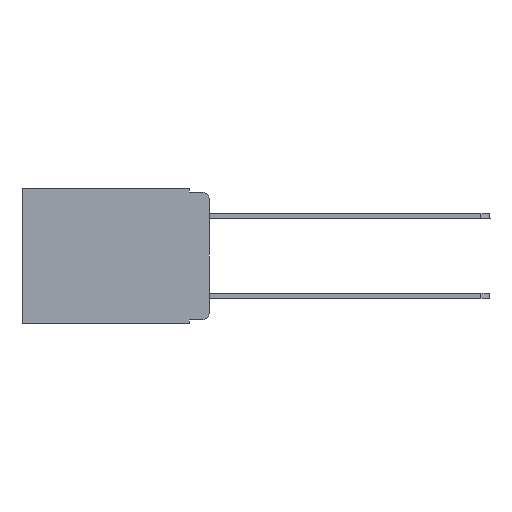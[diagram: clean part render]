
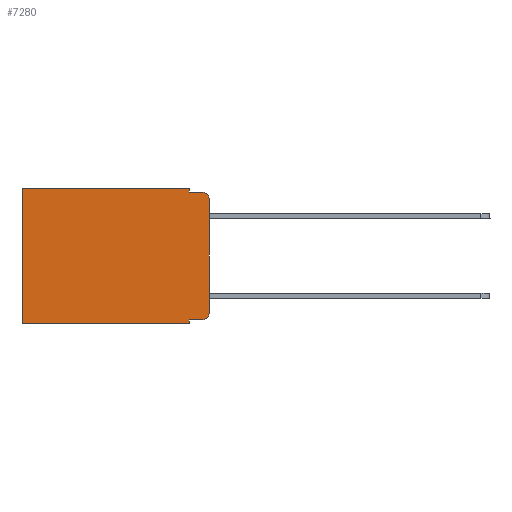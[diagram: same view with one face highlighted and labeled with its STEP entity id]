
A CAD part, left-side view. The second image highlights one B-rep face of the part: STEP entity #7280.
In plain terms, the highlighted planar face has unit normal (-1, 0, 0).
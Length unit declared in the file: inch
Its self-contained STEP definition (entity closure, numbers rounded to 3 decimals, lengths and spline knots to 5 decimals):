
#407 = EDGE_CURVE ( 'NONE', #6526, #16646, #9754, .T. ) ;
#1067 = CARTESIAN_POINT ( 'NONE',  ( 0.298, 0.051, 0. ) ) ;
#1158 = DIRECTION ( 'NONE',  ( 0., 0., -1. ) ) ;
#1186 = CARTESIAN_POINT ( 'NONE',  ( 0.298, 0.02, -0.01 ) ) ;
#1210 = ORIENTED_EDGE ( 'NONE', *, *, #7421, .T. ) ;
#1386 = CIRCLE ( 'NONE', #23051, 0.02 ) ;
#1728 = EDGE_CURVE ( 'NONE', #17078, #16172, #23592, .T. ) ;
#2132 = VERTEX_POINT ( 'NONE', #2365 ) ;
#2365 = CARTESIAN_POINT ( 'NONE',  ( 0.298, 0., -0.313 ) ) ;
#2420 = DIRECTION ( 'NONE',  ( 1., 0., 0. ) ) ;
#2686 = CARTESIAN_POINT ( 'NONE',  ( 0.298, 0., 0. ) ) ;
#2716 = CARTESIAN_POINT ( 'NONE',  ( 0.298, 0.473, 0. ) ) ;
#2943 = AXIS2_PLACEMENT_3D ( 'NONE', #6712, #18607, #1158 ) ;
#2954 = ORIENTED_EDGE ( 'NONE', *, *, #4321, .F. ) ;
#2958 = ORIENTED_EDGE ( 'NONE', *, *, #407, .T. ) ;
#3098 = CARTESIAN_POINT ( 'NONE',  ( 0.298, 0.051, -0.333 ) ) ;
#3185 = ORIENTED_EDGE ( 'NONE', *, *, #10088, .F. ) ;
#3444 = VECTOR ( 'NONE', #9585, 39.37008 ) ;
#3748 = DIRECTION ( 'NONE',  ( 0., 1., 0. ) ) ;
#4321 = EDGE_CURVE ( 'NONE', #12996, #24492, #6177, .T. ) ;
#4470 = DIRECTION ( 'NONE',  ( 0., 0., -1. ) ) ;
#4957 = EDGE_CURVE ( 'NONE', #16172, #10655, #17126, .T. ) ;
#6177 = LINE ( 'NONE', #19108, #12927 ) ;
#6417 = DIRECTION ( 'NONE',  ( 0., 0., -1. ) ) ;
#6509 = CARTESIAN_POINT ( 'NONE',  ( 0.298, 0.02, -0.333 ) ) ;
#6526 = VERTEX_POINT ( 'NONE', #1067 ) ;
#6712 = CARTESIAN_POINT ( 'NONE',  ( 0.298, 0.02, -0.03 ) ) ;
#7280 = ADVANCED_FACE ( 'NONE', ( #8207 ), #16119, .F. ) ;
#7421 = EDGE_CURVE ( 'NONE', #24477, #24492, #21342, .T. ) ;
#8207 = FACE_OUTER_BOUND ( 'NONE', #16740, .T. ) ;
#8949 = VERTEX_POINT ( 'NONE', #6509 ) ;
#9114 = DIRECTION ( 'NONE',  ( 0., -1., 0. ) ) ;
#9568 = VECTOR ( 'NONE', #4470, 39.37008 ) ;
#9585 = DIRECTION ( 'NONE',  ( 0., 1., 0. ) ) ;
#9754 = LINE ( 'NONE', #22705, #18976 ) ;
#10088 = EDGE_CURVE ( 'NONE', #24477, #2132, #15806, .T. ) ;
#10244 = ORIENTED_EDGE ( 'NONE', *, *, #13080, .T. ) ;
#10430 = CARTESIAN_POINT ( 'NONE',  ( 0.298, 0.051, 0. ) ) ;
#10655 = VERTEX_POINT ( 'NONE', #21533 ) ;
#11205 = ORIENTED_EDGE ( 'NONE', *, *, #1728, .F. ) ;
#12122 = VECTOR ( 'NONE', #23179, 39.37008 ) ;
#12878 = ORIENTED_EDGE ( 'NONE', *, *, #19840, .F. ) ;
#12927 = VECTOR ( 'NONE', #15723, 39.37008 ) ;
#12996 = VERTEX_POINT ( 'NONE', #22286 ) ;
#12997 = LINE ( 'NONE', #3098, #23626 ) ;
#13080 = EDGE_CURVE ( 'NONE', #17078, #8949, #12997, .T. ) ;
#13104 = VECTOR ( 'NONE', #6417, 39.37008 ) ;
#13181 = DIRECTION ( 'NONE',  ( 0., 0., -1. ) ) ;
#13551 = CARTESIAN_POINT ( 'NONE',  ( 0.298, 0., 0. ) ) ;
#14868 = VECTOR ( 'NONE', #13181, 39.37008 ) ;
#15123 = EDGE_CURVE ( 'NONE', #8949, #2132, #1386, .T. ) ;
#15324 = CARTESIAN_POINT ( 'NONE',  ( 0.298, 0.051, 0. ) ) ;
#15704 = DIRECTION ( 'NONE',  ( 0., 0., -1. ) ) ;
#15719 = CARTESIAN_POINT ( 'NONE',  ( 0.298, 0., -0.343 ) ) ;
#15723 = DIRECTION ( 'NONE',  ( 0., -1., 0. ) ) ;
#15806 = LINE ( 'NONE', #13551, #12122 ) ;
#16003 = ORIENTED_EDGE ( 'NONE', *, *, #18664, .T. ) ;
#16119 = PLANE ( 'NONE',  #16730 ) ;
#16172 = VERTEX_POINT ( 'NONE', #20262 ) ;
#16646 = VERTEX_POINT ( 'NONE', #18583 ) ;
#16730 = AXIS2_PLACEMENT_3D ( 'NONE', #2686, #2420, #21753 ) ;
#16740 = EDGE_LOOP ( 'NONE', ( #3185, #1210, #2954, #12878, #2958, #16003, #18872, #11205, #10244, #24614 ) ) ;
#17078 = VERTEX_POINT ( 'NONE', #23933 ) ;
#17126 = LINE ( 'NONE', #15719, #3444 ) ;
#18578 = LINE ( 'NONE', #15324, #14868 ) ;
#18583 = CARTESIAN_POINT ( 'NONE',  ( 0.298, 0.473, 0. ) ) ;
#18607 = DIRECTION ( 'NONE',  ( -1., 0., 0. ) ) ;
#18664 = EDGE_CURVE ( 'NONE', #16646, #10655, #19515, .T. ) ;
#18872 = ORIENTED_EDGE ( 'NONE', *, *, #4957, .F. ) ;
#18976 = VECTOR ( 'NONE', #3748, 39.37008 ) ;
#19108 = CARTESIAN_POINT ( 'NONE',  ( 0.298, 0.051, -0.01 ) ) ;
#19515 = LINE ( 'NONE', #2716, #9568 ) ;
#19840 = EDGE_CURVE ( 'NONE', #6526, #12996, #18578, .T. ) ;
#19842 = DIRECTION ( 'NONE',  ( -1., 0., 0. ) ) ;
#20262 = CARTESIAN_POINT ( 'NONE',  ( 0.298, 0.051, -0.343 ) ) ;
#21342 = CIRCLE ( 'NONE', #2943, 0.02 ) ;
#21533 = CARTESIAN_POINT ( 'NONE',  ( 0.298, 0.473, -0.343 ) ) ;
#21753 = DIRECTION ( 'NONE',  ( 0., 0., -1. ) ) ;
#22286 = CARTESIAN_POINT ( 'NONE',  ( 0.298, 0.051, -0.01 ) ) ;
#22705 = CARTESIAN_POINT ( 'NONE',  ( 0.298, 0., 0. ) ) ;
#23051 = AXIS2_PLACEMENT_3D ( 'NONE', #23328, #19842, #15704 ) ;
#23179 = DIRECTION ( 'NONE',  ( 0., 0., -1. ) ) ;
#23328 = CARTESIAN_POINT ( 'NONE',  ( 0.298, 0.02, -0.313 ) ) ;
#23592 = LINE ( 'NONE', #10430, #13104 ) ;
#23626 = VECTOR ( 'NONE', #9114, 39.37008 ) ;
#23933 = CARTESIAN_POINT ( 'NONE',  ( 0.298, 0.051, -0.333 ) ) ;
#24397 = CARTESIAN_POINT ( 'NONE',  ( 0.298, 0., -0.03 ) ) ;
#24477 = VERTEX_POINT ( 'NONE', #24397 ) ;
#24492 = VERTEX_POINT ( 'NONE', #1186 ) ;
#24614 = ORIENTED_EDGE ( 'NONE', *, *, #15123, .T. ) ;
